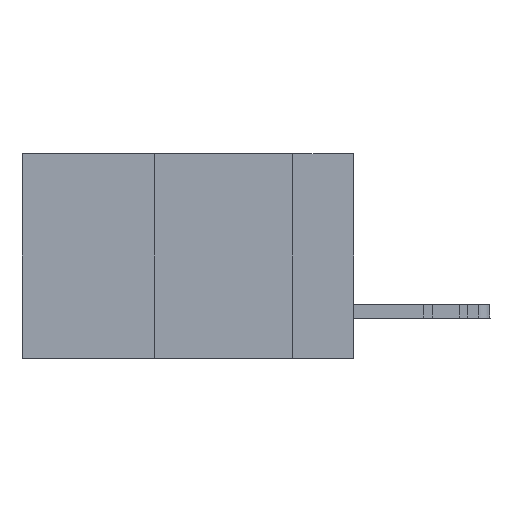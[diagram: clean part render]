
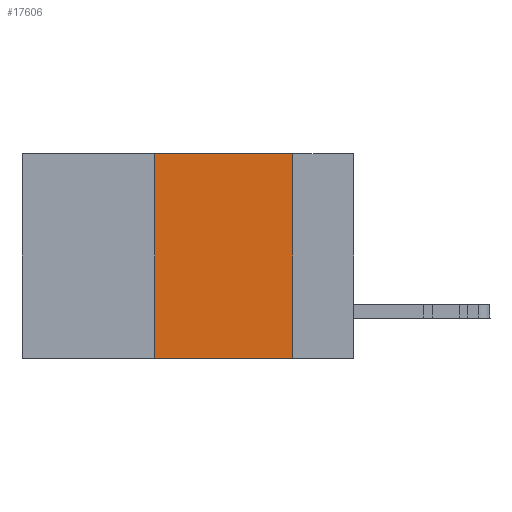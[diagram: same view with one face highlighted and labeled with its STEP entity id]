
A CAD part, left-side view. The second image highlights one B-rep face of the part: STEP entity #17606.
In plain terms, the highlighted planar face has unit normal (-1, 0, 0).
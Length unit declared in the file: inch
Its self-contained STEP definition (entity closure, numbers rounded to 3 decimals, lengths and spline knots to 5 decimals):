
#2636 = DIRECTION ( 'NONE',  ( 0., -1., 0. ) ) ;
#4002 = VECTOR ( 'NONE', #16730, 39.37008 ) ;
#5021 = LINE ( 'NONE', #29822, #4002 ) ;
#5144 = DIRECTION ( 'NONE',  ( 1., 0., 0. ) ) ;
#7699 = VECTOR ( 'NONE', #2636, 39.37008 ) ;
#8918 = EDGE_CURVE ( 'NONE', #16096, #20479, #31697, .T. ) ;
#9588 = ORIENTED_EDGE ( 'NONE', *, *, #38653, .T. ) ;
#11490 = DIRECTION ( 'NONE',  ( 0., 0., -1. ) ) ;
#14216 = DIRECTION ( 'NONE',  ( 0., 0., -1. ) ) ;
#14828 = EDGE_LOOP ( 'NONE', ( #17936, #31153, #25240, #9588 ) ) ;
#15039 = EDGE_CURVE ( 'NONE', #20479, #31915, #34722, .T. ) ;
#15242 = FACE_OUTER_BOUND ( 'NONE', #14828, .T. ) ;
#16096 = VERTEX_POINT ( 'NONE', #23852 ) ;
#16730 = DIRECTION ( 'NONE',  ( 0., -1., 0. ) ) ;
#17555 = VERTEX_POINT ( 'NONE', #36339 ) ;
#17606 = ADVANCED_FACE ( 'NONE', ( #15242 ), #17643, .F. ) ;
#17643 = PLANE ( 'NONE',  #19440 ) ;
#17936 = ORIENTED_EDGE ( 'NONE', *, *, #35625, .F. ) ;
#17969 = VECTOR ( 'NONE', #11490, 39.37008 ) ;
#17979 = CARTESIAN_POINT ( 'NONE',  ( 0., 0.36, 0. ) ) ;
#18560 = CARTESIAN_POINT ( 'NONE',  ( 0., 0.6, 0. ) ) ;
#19440 = AXIS2_PLACEMENT_3D ( 'NONE', #21165, #5144, #14216 ) ;
#20479 = VERTEX_POINT ( 'NONE', #28642 ) ;
#21165 = CARTESIAN_POINT ( 'NONE',  ( 0., 0.6, 0. ) ) ;
#23852 = CARTESIAN_POINT ( 'NONE',  ( 0., 0.36, -0.37 ) ) ;
#25240 = ORIENTED_EDGE ( 'NONE', *, *, #8918, .F. ) ;
#26605 = LINE ( 'NONE', #27848, #17969 ) ;
#27848 = CARTESIAN_POINT ( 'NONE',  ( 0., 0.11, 0. ) ) ;
#28642 = CARTESIAN_POINT ( 'NONE',  ( 0., 0.36, 0. ) ) ;
#29822 = CARTESIAN_POINT ( 'NONE',  ( 0., 0.6, -0.37 ) ) ;
#31153 = ORIENTED_EDGE ( 'NONE', *, *, #15039, .F. ) ;
#31697 = LINE ( 'NONE', #17979, #34772 ) ;
#31915 = VERTEX_POINT ( 'NONE', #33842 ) ;
#33842 = CARTESIAN_POINT ( 'NONE',  ( 0., 0.11, 0. ) ) ;
#34722 = LINE ( 'NONE', #18560, #7699 ) ;
#34772 = VECTOR ( 'NONE', #40305, 39.37008 ) ;
#35625 = EDGE_CURVE ( 'NONE', #31915, #17555, #26605, .T. ) ;
#36339 = CARTESIAN_POINT ( 'NONE',  ( 0., 0.11, -0.37 ) ) ;
#38653 = EDGE_CURVE ( 'NONE', #16096, #17555, #5021, .T. ) ;
#40305 = DIRECTION ( 'NONE',  ( 0., 0., 1. ) ) ;
